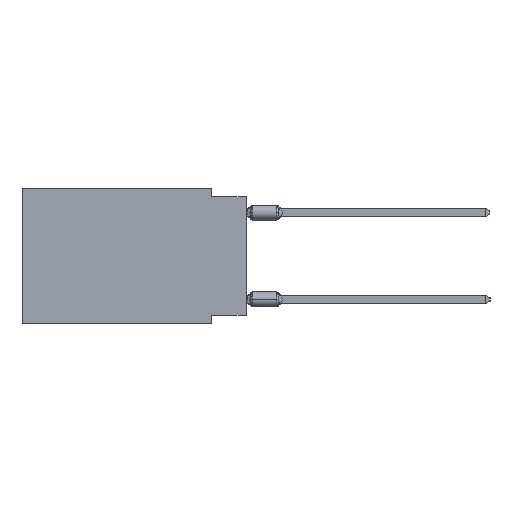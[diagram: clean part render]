
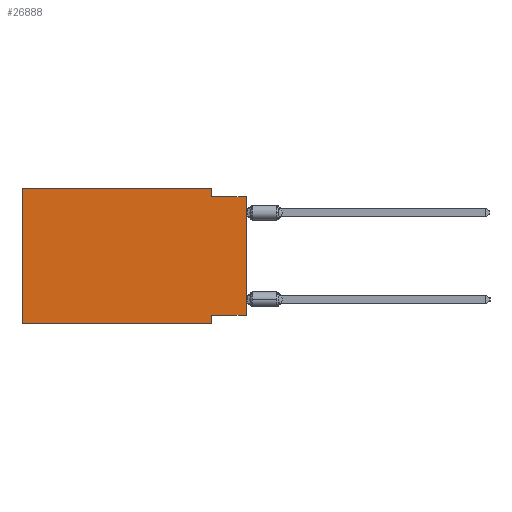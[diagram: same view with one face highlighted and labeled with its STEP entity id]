
A CAD part, left-side view. The second image highlights one B-rep face of the part: STEP entity #26888.
In plain terms, the highlighted planar face has unit normal (-1, 0, 0).
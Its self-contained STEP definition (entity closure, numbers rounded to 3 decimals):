
#299 = CARTESIAN_POINT ( 'NONE',  ( 0., 2.54, -0.635 ) ) ;
#514 = DIRECTION ( 'NONE',  ( 0., 0., 1. ) ) ;
#1188 = ORIENTED_EDGE ( 'NONE', *, *, #38234, .F. ) ;
#1260 = DIRECTION ( 'NONE',  ( 0., 0., 1. ) ) ;
#3197 = CARTESIAN_POINT ( 'NONE',  ( 0., 2.54, 0. ) ) ;
#4170 = DIRECTION ( 'NONE',  ( 0., 1., 0. ) ) ;
#6515 = CARTESIAN_POINT ( 'NONE',  ( 0., 16.383, -9.906 ) ) ;
#6565 = PLANE ( 'NONE',  #44957 ) ;
#7339 = VERTEX_POINT ( 'NONE', #299 ) ;
#7491 = LINE ( 'NONE', #3197, #38883 ) ;
#8081 = EDGE_LOOP ( 'NONE', ( #24467, #53462, #40141, #1188, #28707, #27284, #53174, #8708 ) ) ;
#8465 = VECTOR ( 'NONE', #514, 1000. ) ;
#8708 = ORIENTED_EDGE ( 'NONE', *, *, #44986, .F. ) ;
#10389 = LINE ( 'NONE', #32073, #22251 ) ;
#10399 = CARTESIAN_POINT ( 'NONE',  ( 0., 0., -9.271 ) ) ;
#10539 = EDGE_CURVE ( 'NONE', #37203, #7339, #7491, .T. ) ;
#11110 = DIRECTION ( 'NONE',  ( 0., -1., 0. ) ) ;
#14510 = CARTESIAN_POINT ( 'NONE',  ( 0., 2.54, -9.906 ) ) ;
#14862 = FACE_OUTER_BOUND ( 'NONE', #8081, .T. ) ;
#17802 = VERTEX_POINT ( 'NONE', #10399 ) ;
#18931 = EDGE_CURVE ( 'NONE', #17802, #26857, #26465, .T. ) ;
#18945 = LINE ( 'NONE', #54607, #55134 ) ;
#19448 = LINE ( 'NONE', #36007, #40766 ) ;
#19688 = CARTESIAN_POINT ( 'NONE',  ( 0., 0., -0.635 ) ) ;
#20228 = CARTESIAN_POINT ( 'NONE',  ( 0., 16.383, 0. ) ) ;
#21886 = DIRECTION ( 'NONE',  ( 0., -1., 0. ) ) ;
#22047 = EDGE_CURVE ( 'NONE', #48332, #32217, #10389, .T. ) ;
#22251 = VECTOR ( 'NONE', #1260, 1000. ) ;
#23167 = EDGE_CURVE ( 'NONE', #33968, #49831, #18945, .T. ) ;
#24176 = EDGE_CURVE ( 'NONE', #7339, #26857, #25060, .T. ) ;
#24467 = ORIENTED_EDGE ( 'NONE', *, *, #18931, .T. ) ;
#25060 = LINE ( 'NONE', #51036, #40221 ) ;
#25849 = LINE ( 'NONE', #43268, #53915 ) ;
#26465 = LINE ( 'NONE', #39611, #8465 ) ;
#26857 = VERTEX_POINT ( 'NONE', #19688 ) ;
#26888 = ADVANCED_FACE ( 'NONE', ( #14862 ), #6565, .F. ) ;
#27284 = ORIENTED_EDGE ( 'NONE', *, *, #39048, .T. ) ;
#28707 = ORIENTED_EDGE ( 'NONE', *, *, #22047, .F. ) ;
#32073 = CARTESIAN_POINT ( 'NONE',  ( 0., 16.383, 0. ) ) ;
#32217 = VERTEX_POINT ( 'NONE', #20228 ) ;
#32369 = DIRECTION ( 'NONE',  ( 0., 0., -1. ) ) ;
#33656 = CARTESIAN_POINT ( 'NONE',  ( 0., 16.383, 0. ) ) ;
#33968 = VERTEX_POINT ( 'NONE', #34181 ) ;
#34181 = CARTESIAN_POINT ( 'NONE',  ( 0., 2.54, -9.271 ) ) ;
#36007 = CARTESIAN_POINT ( 'NONE',  ( 0., 16.383, 0. ) ) ;
#37203 = VERTEX_POINT ( 'NONE', #41313 ) ;
#38234 = EDGE_CURVE ( 'NONE', #32217, #37203, #19448, .T. ) ;
#38883 = VECTOR ( 'NONE', #43684, 1000. ) ;
#39032 = LINE ( 'NONE', #47878, #49077 ) ;
#39048 = EDGE_CURVE ( 'NONE', #48332, #49831, #39032, .T. ) ;
#39611 = CARTESIAN_POINT ( 'NONE',  ( 0., 0., 0. ) ) ;
#40141 = ORIENTED_EDGE ( 'NONE', *, *, #10539, .F. ) ;
#40221 = VECTOR ( 'NONE', #11110, 1000. ) ;
#40766 = VECTOR ( 'NONE', #44284, 1000. ) ;
#41313 = CARTESIAN_POINT ( 'NONE',  ( 0., 2.54, 0. ) ) ;
#43268 = CARTESIAN_POINT ( 'NONE',  ( 0., 0., -9.271 ) ) ;
#43684 = DIRECTION ( 'NONE',  ( 0., 0., -1. ) ) ;
#44284 = DIRECTION ( 'NONE',  ( 0., -1., 0. ) ) ;
#44957 = AXIS2_PLACEMENT_3D ( 'NONE', #33656, #55906, #51624 ) ;
#44986 = EDGE_CURVE ( 'NONE', #17802, #33968, #25849, .T. ) ;
#47878 = CARTESIAN_POINT ( 'NONE',  ( 0., 16.383, -9.906 ) ) ;
#48332 = VERTEX_POINT ( 'NONE', #6515 ) ;
#49077 = VECTOR ( 'NONE', #21886, 1000. ) ;
#49831 = VERTEX_POINT ( 'NONE', #14510 ) ;
#51036 = CARTESIAN_POINT ( 'NONE',  ( 0., 0., -0.635 ) ) ;
#51624 = DIRECTION ( 'NONE',  ( 0., 0., -1. ) ) ;
#53174 = ORIENTED_EDGE ( 'NONE', *, *, #23167, .F. ) ;
#53462 = ORIENTED_EDGE ( 'NONE', *, *, #24176, .F. ) ;
#53915 = VECTOR ( 'NONE', #4170, 1000. ) ;
#54607 = CARTESIAN_POINT ( 'NONE',  ( 0., 2.54, -9.906 ) ) ;
#55134 = VECTOR ( 'NONE', #32369, 1000. ) ;
#55906 = DIRECTION ( 'NONE',  ( 1., 0., 0. ) ) ;
